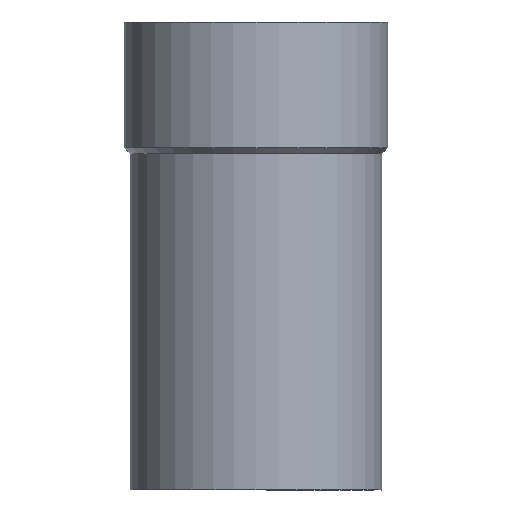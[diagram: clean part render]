
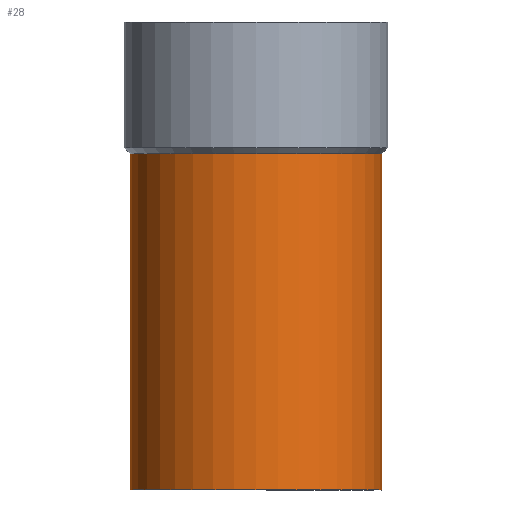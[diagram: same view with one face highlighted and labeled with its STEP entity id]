
A CAD part, left-side view. The second image highlights one B-rep face of the part: STEP entity #28.
In plain terms, the highlighted cylindrical face has radius 27.305 mm (diameter 54.61 mm), a partial arc.
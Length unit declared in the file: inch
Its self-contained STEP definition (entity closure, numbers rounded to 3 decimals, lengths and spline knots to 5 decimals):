
#8 = ORIENTED_EDGE ( 'NONE', *, *, #2490, .F. ) ;
#28 = ADVANCED_FACE ( 'NONE', ( #3347 ), #1665, .T. ) ;
#34 = AXIS2_PLACEMENT_3D ( 'NONE', #987, #3036, #3022 ) ;
#229 = DIRECTION ( 'NONE',  ( 0., 0., -1. ) ) ;
#622 = VERTEX_POINT ( 'NONE', #1715 ) ;
#661 = EDGE_LOOP ( 'NONE', ( #8, #3130, #1439, #2051 ) ) ;
#932 = VECTOR ( 'NONE', #2920, 39.37008 ) ;
#987 = CARTESIAN_POINT ( 'NONE',  ( 0., 0., 0. ) ) ;
#1013 = EDGE_CURVE ( 'NONE', #2185, #2243, #3344, .T. ) ;
#1015 = CARTESIAN_POINT ( 'NONE',  ( 0., 1.075, 2.875 ) ) ;
#1069 = CARTESIAN_POINT ( 'NONE',  ( 0., 1.075, 0. ) ) ;
#1213 = AXIS2_PLACEMENT_3D ( 'NONE', #3378, #3070, #3367 ) ;
#1240 = CARTESIAN_POINT ( 'NONE',  ( 0., -1.075, 0. ) ) ;
#1295 = EDGE_CURVE ( 'NONE', #1719, #2243, #3209, .T. ) ;
#1439 = ORIENTED_EDGE ( 'NONE', *, *, #1013, .T. ) ;
#1642 = DIRECTION ( 'NONE',  ( 0., 1., 0. ) ) ;
#1665 = CYLINDRICAL_SURFACE ( 'NONE', #2116, 1.075 ) ;
#1715 = CARTESIAN_POINT ( 'NONE',  ( 0., -1.075, 2.875 ) ) ;
#1719 = VERTEX_POINT ( 'NONE', #1240 ) ;
#1821 = DIRECTION ( 'NONE',  ( 0., 0., -1. ) ) ;
#2051 = ORIENTED_EDGE ( 'NONE', *, *, #1295, .F. ) ;
#2111 = CARTESIAN_POINT ( 'NONE',  ( 0., -1.075, 0. ) ) ;
#2116 = AXIS2_PLACEMENT_3D ( 'NONE', #3778, #229, #1642 ) ;
#2185 = VERTEX_POINT ( 'NONE', #1015 ) ;
#2243 = VERTEX_POINT ( 'NONE', #1069 ) ;
#2326 = CARTESIAN_POINT ( 'NONE',  ( 0., 1.075, 0. ) ) ;
#2490 = EDGE_CURVE ( 'NONE', #622, #1719, #2881, .T. ) ;
#2881 = LINE ( 'NONE', #2111, #3482 ) ;
#2920 = DIRECTION ( 'NONE',  ( 0., 0., -1. ) ) ;
#2922 = EDGE_CURVE ( 'NONE', #2185, #622, #3203, .T. ) ;
#3022 = DIRECTION ( 'NONE',  ( 0., 1., 0. ) ) ;
#3036 = DIRECTION ( 'NONE',  ( 0., 0., -1. ) ) ;
#3070 = DIRECTION ( 'NONE',  ( 0., 0., 1. ) ) ;
#3130 = ORIENTED_EDGE ( 'NONE', *, *, #2922, .F. ) ;
#3203 = CIRCLE ( 'NONE', #1213, 1.075 ) ;
#3209 = CIRCLE ( 'NONE', #34, 1.075 ) ;
#3344 = LINE ( 'NONE', #2326, #932 ) ;
#3347 = FACE_OUTER_BOUND ( 'NONE', #661, .T. ) ;
#3367 = DIRECTION ( 'NONE',  ( 0., -1., 0. ) ) ;
#3378 = CARTESIAN_POINT ( 'NONE',  ( 0., 0., 2.875 ) ) ;
#3482 = VECTOR ( 'NONE', #1821, 39.37008 ) ;
#3778 = CARTESIAN_POINT ( 'NONE',  ( 0., 0., 0. ) ) ;
